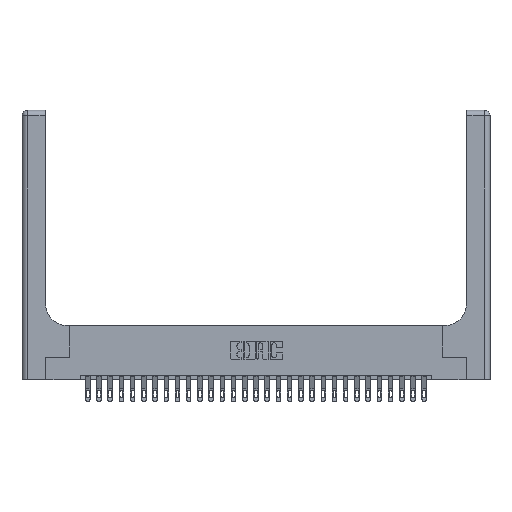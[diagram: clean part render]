
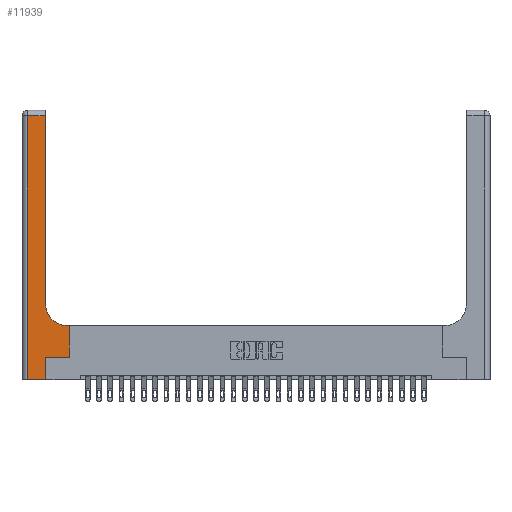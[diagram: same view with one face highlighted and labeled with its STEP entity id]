
A CAD part, top view. The second image highlights one B-rep face of the part: STEP entity #11939.
In plain terms, the highlighted planar face has unit normal (0, 0, 1).
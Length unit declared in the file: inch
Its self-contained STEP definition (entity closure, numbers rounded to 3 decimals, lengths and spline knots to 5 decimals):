
#133 = PLANE ( 'NONE',  #13422 ) ;
#227 = DIRECTION ( 'NONE',  ( 0., 0., -1. ) ) ;
#346 = DIRECTION ( 'NONE',  ( 0., 1., 0. ) ) ;
#935 = VECTOR ( 'NONE', #5792, 39.37008 ) ;
#1482 = CARTESIAN_POINT ( 'NONE',  ( 0.265, 0.25, 0.37 ) ) ;
#1543 = VECTOR ( 'NONE', #6487, 39.37008 ) ;
#1580 = VECTOR ( 'NONE', #346, 39.37008 ) ;
#1870 = EDGE_CURVE ( 'NONE', #22687, #19989, #19091, .T. ) ;
#2057 = ORIENTED_EDGE ( 'NONE', *, *, #3309, .T. ) ;
#2142 = CARTESIAN_POINT ( 'NONE',  ( 0.265, 0., 0.37 ) ) ;
#2376 = ORIENTED_EDGE ( 'NONE', *, *, #1870, .T. ) ;
#2566 = ORIENTED_EDGE ( 'NONE', *, *, #8631, .T. ) ;
#2820 = VERTEX_POINT ( 'NONE', #5739 ) ;
#2995 = EDGE_CURVE ( 'NONE', #11872, #21888, #3504, .T. ) ;
#3056 = VECTOR ( 'NONE', #27176, 39.37008 ) ;
#3309 = EDGE_CURVE ( 'NONE', #22569, #19296, #12431, .T. ) ;
#3504 = LINE ( 'NONE', #25565, #1580 ) ;
#3604 = CARTESIAN_POINT ( 'NONE',  ( 0.06, 3., 0.37 ) ) ;
#4013 = DIRECTION ( 'NONE',  ( 1., 0., 0. ) ) ;
#4823 = CARTESIAN_POINT ( 'NONE',  ( 0.26, 0.6, 0.37 ) ) ;
#5402 = CARTESIAN_POINT ( 'NONE',  ( 0., 2.94, 0.37 ) ) ;
#5739 = CARTESIAN_POINT ( 'NONE',  ( 0.51, 0.6, 0.37 ) ) ;
#5792 = DIRECTION ( 'NONE',  ( 0., 1., 0. ) ) ;
#6054 = LINE ( 'NONE', #4823, #19975 ) ;
#6129 = DIRECTION ( 'NONE',  ( 0., 0., -1. ) ) ;
#6460 = DIRECTION ( 'NONE',  ( -1., 0., 0. ) ) ;
#6487 = DIRECTION ( 'NONE',  ( -1., 0., 0. ) ) ;
#7310 = VECTOR ( 'NONE', #22083, 39.37008 ) ;
#7732 = CARTESIAN_POINT ( 'NONE',  ( 0.26, 3., 0.37 ) ) ;
#8631 = EDGE_CURVE ( 'NONE', #21888, #15745, #12954, .T. ) ;
#9478 = VECTOR ( 'NONE', #20863, 39.37008 ) ;
#10375 = AXIS2_PLACEMENT_3D ( 'NONE', #14453, #6129, #4013 ) ;
#10376 = ORIENTED_EDGE ( 'NONE', *, *, #11183, .T. ) ;
#10997 = EDGE_LOOP ( 'NONE', ( #2376, #16598, #2057, #14108, #24642, #2566, #14932, #17911, #10376 ) ) ;
#11120 = LINE ( 'NONE', #15718, #11768 ) ;
#11183 = EDGE_CURVE ( 'NONE', #2820, #22687, #25659, .T. ) ;
#11459 = CARTESIAN_POINT ( 'NONE',  ( 0.528, 0.25, 0.37 ) ) ;
#11768 = VECTOR ( 'NONE', #26293, 39.37008 ) ;
#11872 = VERTEX_POINT ( 'NONE', #2142 ) ;
#11939 = ADVANCED_FACE ( 'NONE', ( #13739 ), #133, .F. ) ;
#12431 = LINE ( 'NONE', #3604, #9478 ) ;
#12954 = LINE ( 'NONE', #21048, #3056 ) ;
#13422 = AXIS2_PLACEMENT_3D ( 'NONE', #21316, #227, #6460 ) ;
#13739 = FACE_OUTER_BOUND ( 'NONE', #10997, .T. ) ;
#14108 = ORIENTED_EDGE ( 'NONE', *, *, #23822, .T. ) ;
#14173 = EDGE_CURVE ( 'NONE', #23573, #2820, #6054, .T. ) ;
#14453 = CARTESIAN_POINT ( 'NONE',  ( 0.51, 0.85, 0.37 ) ) ;
#14472 = CARTESIAN_POINT ( 'NONE',  ( 0.06, 0., 0.37 ) ) ;
#14932 = ORIENTED_EDGE ( 'NONE', *, *, #26822, .T. ) ;
#15718 = CARTESIAN_POINT ( 'NONE',  ( 0.528, 0.25, 0.37 ) ) ;
#15745 = VERTEX_POINT ( 'NONE', #11459 ) ;
#16598 = ORIENTED_EDGE ( 'NONE', *, *, #20775, .T. ) ;
#16645 = CARTESIAN_POINT ( 'NONE',  ( 0.26, 2.94, 0.37 ) ) ;
#17015 = CARTESIAN_POINT ( 'NONE',  ( 0.528, 0.6, 0.37 ) ) ;
#17911 = ORIENTED_EDGE ( 'NONE', *, *, #14173, .T. ) ;
#18779 = CARTESIAN_POINT ( 'NONE',  ( 0.06, 2.94, 0.37 ) ) ;
#19091 = LINE ( 'NONE', #7732, #935 ) ;
#19296 = VERTEX_POINT ( 'NONE', #14472 ) ;
#19583 = LINE ( 'NONE', #20176, #7310 ) ;
#19975 = VECTOR ( 'NONE', #21801, 39.37008 ) ;
#19989 = VERTEX_POINT ( 'NONE', #16645 ) ;
#20176 = CARTESIAN_POINT ( 'NONE',  ( 0., 0., 0.37 ) ) ;
#20775 = EDGE_CURVE ( 'NONE', #19989, #22569, #26587, .T. ) ;
#20863 = DIRECTION ( 'NONE',  ( 0., -1., 0. ) ) ;
#21048 = CARTESIAN_POINT ( 'NONE',  ( 0.265, 0.25, 0.37 ) ) ;
#21316 = CARTESIAN_POINT ( 'NONE',  ( 0., 3., 0.37 ) ) ;
#21724 = CARTESIAN_POINT ( 'NONE',  ( 0.26, 0.85, 0.37 ) ) ;
#21801 = DIRECTION ( 'NONE',  ( -1., 0., 0. ) ) ;
#21888 = VERTEX_POINT ( 'NONE', #1482 ) ;
#22083 = DIRECTION ( 'NONE',  ( 1., 0., 0. ) ) ;
#22569 = VERTEX_POINT ( 'NONE', #18779 ) ;
#22687 = VERTEX_POINT ( 'NONE', #21724 ) ;
#23573 = VERTEX_POINT ( 'NONE', #17015 ) ;
#23822 = EDGE_CURVE ( 'NONE', #19296, #11872, #19583, .T. ) ;
#24642 = ORIENTED_EDGE ( 'NONE', *, *, #2995, .T. ) ;
#25565 = CARTESIAN_POINT ( 'NONE',  ( 0.265, 0., 0.37 ) ) ;
#25659 = CIRCLE ( 'NONE', #10375, 0.25 ) ;
#26293 = DIRECTION ( 'NONE',  ( 0., 1., 0. ) ) ;
#26587 = LINE ( 'NONE', #5402, #1543 ) ;
#26822 = EDGE_CURVE ( 'NONE', #15745, #23573, #11120, .T. ) ;
#27176 = DIRECTION ( 'NONE',  ( 1., 0., 0. ) ) ;
